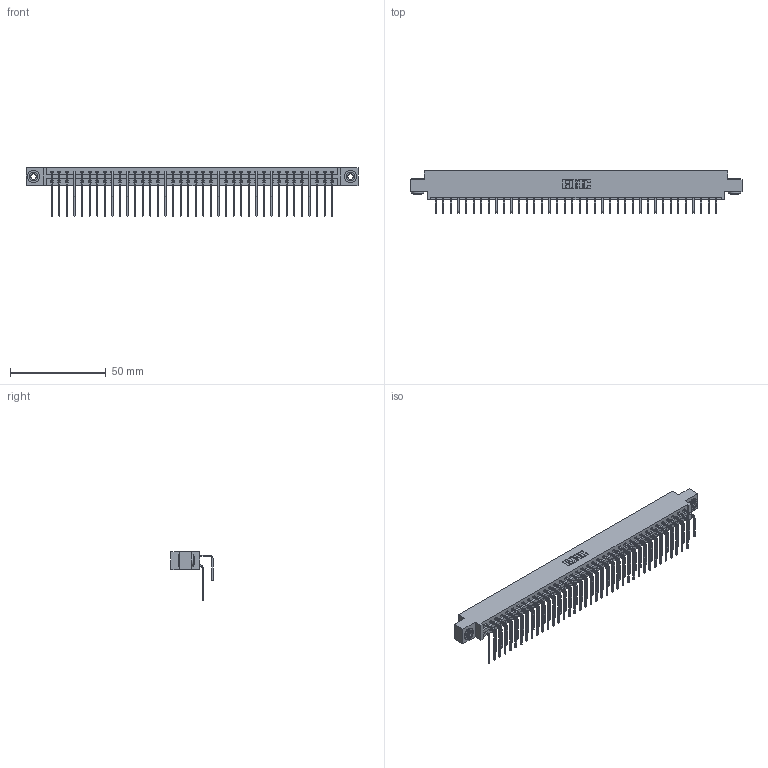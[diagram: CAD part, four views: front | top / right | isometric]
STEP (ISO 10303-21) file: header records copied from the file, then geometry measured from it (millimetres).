
FILE_DESCRIPTION (( 'STEP AP203' ), '1' );
FILE_NAME ('387-076-558-803.STEP', '2019-10-22T04:38:33', ( '' ), ( '' ), 'SwSTEP 2.0', 'SolidWorks 2016', '' );
FILE_SCHEMA (( 'CONFIG_CONTROL_DESIGN' ));
Length unit declared in the file: inch
Products named in the file (5): 345-292-001_558 Tail - 2; 387-076-558-803; 345-292-001_558 559 Tail - 1; 337 Part_0.170 Offset - 0.156 Dia-TH; 345-250-002_345-250-002-102
Assembly tree (79 placements, depth 2):
  387-076-558-803
    337 Part_0.170 Offset - 0.156 Dia-TH
    345-292-001_558 559 Tail - 1  x38
    345-292-001_558 Tail - 2  x38
    345-250-002_345-250-002-102  x2
Bounding box: 173.58 x 22.17 x 25.53 mm (x, y, z)
Volume: 18580.7 mm3; surface area: 23500.3 mm2
Topology: 79 solids, 79 shells, 4412 faces, 13091 edges, 8622 vertices
Faces by surface type: plane 3124, cylinder 1280, cone 8
Entity records: 32546 total; most frequent: CARTESIAN_POINT 5508, ORIENTED_EDGE 5386, DIRECTION 4707, EDGE_CURVE 2693, LINE 2501, VECTOR 2501, VERTEX_POINT 1790, AXIS2_PLACEMENT_3D 1103
